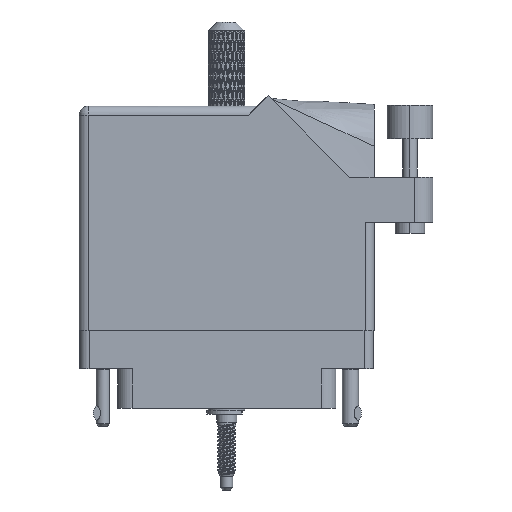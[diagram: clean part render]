
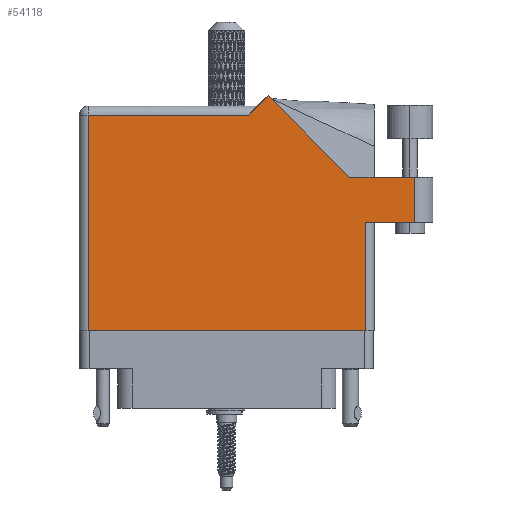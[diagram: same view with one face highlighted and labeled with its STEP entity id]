
A CAD part, front view. The second image highlights one B-rep face of the part: STEP entity #54118.
In plain terms, the highlighted face is planar.
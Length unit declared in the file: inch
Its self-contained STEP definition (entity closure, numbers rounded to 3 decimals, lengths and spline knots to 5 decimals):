
#1811 = AXIS2_PLACEMENT_3D ( 'NONE', #57860, #94144, #50340 ) ;
#3196 = ORIENTED_EDGE ( 'NONE', *, *, #25196, .T. ) ;
#3927 = ORIENTED_EDGE ( 'NONE', *, *, #56528, .T. ) ;
#4126 = VERTEX_POINT ( 'NONE', #93908 ) ;
#5191 = ORIENTED_EDGE ( 'NONE', *, *, #20867, .T. ) ;
#5776 = LINE ( 'NONE', #39235, #64855 ) ;
#7000 = DIRECTION ( 'NONE',  ( -1., 0., 0. ) ) ;
#8249 = LINE ( 'NONE', #95299, #47047 ) ;
#11113 = CARTESIAN_POINT ( 'NONE',  ( 1.84442, 1.044, 0. ) ) ;
#12893 = PLANE ( 'NONE',  #1811 ) ;
#15743 = DIRECTION ( 'NONE',  ( -1., 0., 0. ) ) ;
#17430 = EDGE_CURVE ( 'NONE', #30738, #82732, #5776, .T. ) ;
#19849 = DIRECTION ( 'NONE',  ( -0.707, 0.707, 0. ) ) ;
#20867 = EDGE_CURVE ( 'NONE', #4126, #28562, #59453, .T. ) ;
#21137 = ORIENTED_EDGE ( 'NONE', *, *, #63846, .T. ) ;
#25196 = EDGE_CURVE ( 'NONE', #34271, #4126, #103298, .T. ) ;
#25240 = CARTESIAN_POINT ( 'NONE',  ( 1.948, 0.737, 0. ) ) ;
#28098 = LINE ( 'NONE', #98392, #42235 ) ;
#28381 = CARTESIAN_POINT ( 'NONE',  ( 2.285, 1.044, 0. ) ) ;
#28562 = VERTEX_POINT ( 'NONE', #33523 ) ;
#29009 = VECTOR ( 'NONE', #19849, 39.37008 ) ;
#29074 = LINE ( 'NONE', #48620, #29009 ) ;
#30738 = VERTEX_POINT ( 'NONE', #25240 ) ;
#31101 = CARTESIAN_POINT ( 'NONE',  ( 1.948, 0.737, 0. ) ) ;
#33523 = CARTESIAN_POINT ( 'NONE',  ( 0.062, 0., 0. ) ) ;
#33538 = EDGE_CURVE ( 'NONE', #113206, #34271, #102796, .T. ) ;
#34271 = VERTEX_POINT ( 'NONE', #97685 ) ;
#35607 = DIRECTION ( 'NONE',  ( 1., 0., 0. ) ) ;
#35932 = CARTESIAN_POINT ( 'NONE',  ( 2.285, 0.737, 0. ) ) ;
#39235 = CARTESIAN_POINT ( 'NONE',  ( 2.01, 0.737, 0. ) ) ;
#40325 = VERTEX_POINT ( 'NONE', #28381 ) ;
#41109 = DIRECTION ( 'NONE',  ( -0.707, -0.707, 0. ) ) ;
#42235 = VECTOR ( 'NONE', #35607, 39.37008 ) ;
#43451 = LINE ( 'NONE', #78618, #89191 ) ;
#43935 = CARTESIAN_POINT ( 'NONE',  ( 1.28771, 1.60071, 0. ) ) ;
#45126 = VECTOR ( 'NONE', #41109, 39.37008 ) ;
#47047 = VECTOR ( 'NONE', #15743, 39.37008 ) ;
#48136 = CARTESIAN_POINT ( 'NONE',  ( 1.948, 0., 0. ) ) ;
#48620 = CARTESIAN_POINT ( 'NONE',  ( 1.84442, 1.044, 0. ) ) ;
#50241 = CARTESIAN_POINT ( 'NONE',  ( 0., 1.468, 0. ) ) ;
#50340 = DIRECTION ( 'NONE',  ( -1., 0., 0. ) ) ;
#53333 = VECTOR ( 'NONE', #101983, 39.37008 ) ;
#54118 = ADVANCED_FACE ( 'NONE', ( #83797 ), #12893, .F. ) ;
#56528 = EDGE_CURVE ( 'NONE', #40325, #82705, #8249, .T. ) ;
#56745 = ORIENTED_EDGE ( 'NONE', *, *, #33538, .T. ) ;
#57860 = CARTESIAN_POINT ( 'NONE',  ( 0., 1.53, 0. ) ) ;
#59453 = LINE ( 'NONE', #92900, #111893 ) ;
#62139 = EDGE_CURVE ( 'NONE', #82732, #40325, #43451, .T. ) ;
#63458 = ORIENTED_EDGE ( 'NONE', *, *, #62139, .T. ) ;
#63713 = ORIENTED_EDGE ( 'NONE', *, *, #99116, .T. ) ;
#63846 = EDGE_CURVE ( 'NONE', #82705, #113206, #29074, .T. ) ;
#64855 = VECTOR ( 'NONE', #74392, 39.37008 ) ;
#74392 = DIRECTION ( 'NONE',  ( 1., 0., 0. ) ) ;
#75117 = CARTESIAN_POINT ( 'NONE',  ( 1.217, 1.53, 0. ) ) ;
#78618 = CARTESIAN_POINT ( 'NONE',  ( 2.285, 1.044, 0. ) ) ;
#80607 = VECTOR ( 'NONE', #7000, 39.37008 ) ;
#82705 = VERTEX_POINT ( 'NONE', #11113 ) ;
#82732 = VERTEX_POINT ( 'NONE', #35932 ) ;
#83797 = FACE_OUTER_BOUND ( 'NONE', #95257, .T. ) ;
#89191 = VECTOR ( 'NONE', #97022, 39.37008 ) ;
#91605 = LINE ( 'NONE', #31101, #53333 ) ;
#92127 = ORIENTED_EDGE ( 'NONE', *, *, #98568, .T. ) ;
#92900 = CARTESIAN_POINT ( 'NONE',  ( 0.062, 0., 0. ) ) ;
#93464 = DIRECTION ( 'NONE',  ( 0., -1., 0. ) ) ;
#93908 = CARTESIAN_POINT ( 'NONE',  ( 0.062, 1.468, 0. ) ) ;
#94144 = DIRECTION ( 'NONE',  ( 0., 0., -1. ) ) ;
#95257 = EDGE_LOOP ( 'NONE', ( #98738, #63458, #3927, #21137, #56745, #3196, #5191, #92127, #63713 ) ) ;
#95299 = CARTESIAN_POINT ( 'NONE',  ( 2.41, 1.044, 0. ) ) ;
#95904 = VERTEX_POINT ( 'NONE', #48136 ) ;
#97022 = DIRECTION ( 'NONE',  ( 0., 1., 0. ) ) ;
#97685 = CARTESIAN_POINT ( 'NONE',  ( 1.155, 1.468, 0. ) ) ;
#98392 = CARTESIAN_POINT ( 'NONE',  ( 0., 0., 0. ) ) ;
#98568 = EDGE_CURVE ( 'NONE', #28562, #95904, #28098, .T. ) ;
#98738 = ORIENTED_EDGE ( 'NONE', *, *, #17430, .T. ) ;
#99116 = EDGE_CURVE ( 'NONE', #95904, #30738, #91605, .T. ) ;
#101983 = DIRECTION ( 'NONE',  ( 0., 1., 0. ) ) ;
#102796 = LINE ( 'NONE', #75117, #45126 ) ;
#103298 = LINE ( 'NONE', #50241, #80607 ) ;
#111893 = VECTOR ( 'NONE', #93464, 39.37008 ) ;
#113206 = VERTEX_POINT ( 'NONE', #43935 ) ;
